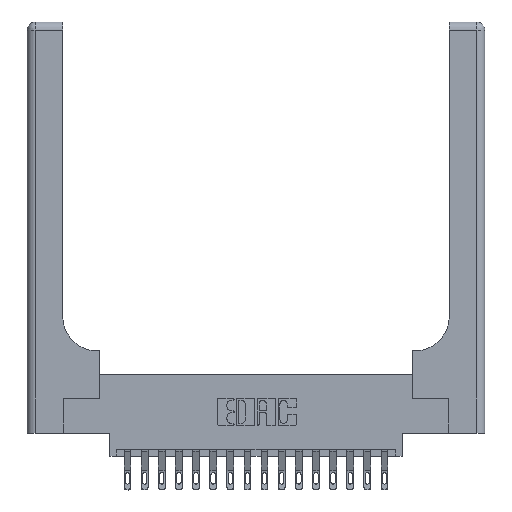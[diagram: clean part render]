
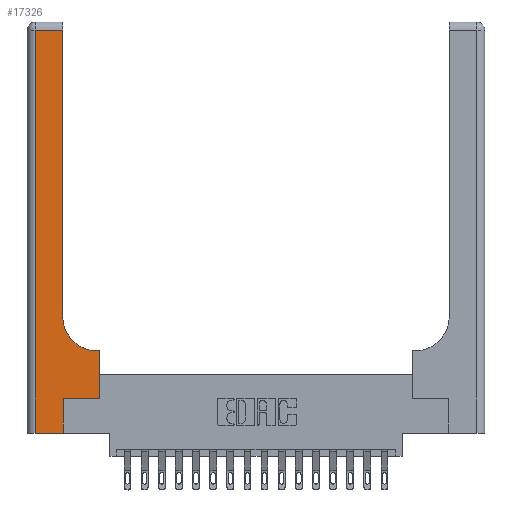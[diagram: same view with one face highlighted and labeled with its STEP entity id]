
A CAD part, top view. The second image highlights one B-rep face of the part: STEP entity #17326.
In plain terms, the highlighted planar face has unit normal (0, 0, 1).
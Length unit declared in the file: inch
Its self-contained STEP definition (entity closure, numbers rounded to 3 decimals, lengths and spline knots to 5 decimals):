
#51 = LINE ( 'NONE', #6856, #16189 ) ;
#417 = ORIENTED_EDGE ( 'NONE', *, *, #19441, .T. ) ;
#775 = EDGE_CURVE ( 'NONE', #4348, #18206, #16440, .T. ) ;
#969 = EDGE_CURVE ( 'NONE', #7376, #7418, #8162, .T. ) ;
#982 = EDGE_LOOP ( 'NONE', ( #9656, #7684, #10253, #3017, #5824, #18833, #3794, #417, #2319 ) ) ;
#1129 = LINE ( 'NONE', #6979, #4694 ) ;
#1224 = DIRECTION ( 'NONE',  ( 0., 0., -1. ) ) ;
#1258 = CARTESIAN_POINT ( 'NONE',  ( 0.528, 0.6, 0.37 ) ) ;
#1745 = EDGE_CURVE ( 'NONE', #18206, #7376, #11112, .T. ) ;
#1883 = DIRECTION ( 'NONE',  ( 1., 0., 0. ) ) ;
#2319 = ORIENTED_EDGE ( 'NONE', *, *, #7392, .T. ) ;
#2387 = VERTEX_POINT ( 'NONE', #19251 ) ;
#2564 = CARTESIAN_POINT ( 'NONE',  ( 0.06, 0., 0.37 ) ) ;
#2622 = LINE ( 'NONE', #18035, #18233 ) ;
#2755 = PLANE ( 'NONE',  #16710 ) ;
#2839 = FACE_OUTER_BOUND ( 'NONE', #982, .T. ) ;
#3017 = ORIENTED_EDGE ( 'NONE', *, *, #775, .T. ) ;
#3207 = DIRECTION ( 'NONE',  ( 0., 1., 0. ) ) ;
#3646 = CARTESIAN_POINT ( 'NONE',  ( 0.265, 0., 0.37 ) ) ;
#3794 = ORIENTED_EDGE ( 'NONE', *, *, #7084, .T. ) ;
#4286 = CARTESIAN_POINT ( 'NONE',  ( 0., 3., 0.37 ) ) ;
#4348 = VERTEX_POINT ( 'NONE', #2564 ) ;
#4694 = VECTOR ( 'NONE', #11569, 39.37008 ) ;
#4829 = EDGE_CURVE ( 'NONE', #9196, #4348, #51, .T. ) ;
#5149 = CARTESIAN_POINT ( 'NONE',  ( 0.51, 0.85, 0.37 ) ) ;
#5661 = CARTESIAN_POINT ( 'NONE',  ( 0.265, 0., 0.37 ) ) ;
#5823 = DIRECTION ( 'NONE',  ( -1., 0., 0. ) ) ;
#5824 = ORIENTED_EDGE ( 'NONE', *, *, #1745, .T. ) ;
#5871 = CARTESIAN_POINT ( 'NONE',  ( 0.06, 2.94, 0.37 ) ) ;
#6522 = CARTESIAN_POINT ( 'NONE',  ( 0.51, 0.6, 0.37 ) ) ;
#6675 = DIRECTION ( 'NONE',  ( 1., 0., 0. ) ) ;
#6856 = CARTESIAN_POINT ( 'NONE',  ( 0.06, 3., 0.37 ) ) ;
#6979 = CARTESIAN_POINT ( 'NONE',  ( 0.26, 0.6, 0.37 ) ) ;
#7084 = EDGE_CURVE ( 'NONE', #7418, #9750, #2622, .T. ) ;
#7252 = CARTESIAN_POINT ( 'NONE',  ( 0., 2.94, 0.37 ) ) ;
#7376 = VERTEX_POINT ( 'NONE', #12654 ) ;
#7392 = EDGE_CURVE ( 'NONE', #11188, #11655, #17981, .T. ) ;
#7418 = VERTEX_POINT ( 'NONE', #11252 ) ;
#7596 = LINE ( 'NONE', #15277, #15171 ) ;
#7684 = ORIENTED_EDGE ( 'NONE', *, *, #17955, .T. ) ;
#7954 = CARTESIAN_POINT ( 'NONE',  ( 0., 0., 0.37 ) ) ;
#8162 = LINE ( 'NONE', #17450, #15729 ) ;
#8340 = VECTOR ( 'NONE', #19336, 39.37008 ) ;
#9196 = VERTEX_POINT ( 'NONE', #5871 ) ;
#9656 = ORIENTED_EDGE ( 'NONE', *, *, #17540, .T. ) ;
#9750 = VERTEX_POINT ( 'NONE', #1258 ) ;
#9940 = DIRECTION ( 'NONE',  ( 1., 0., 0. ) ) ;
#10253 = ORIENTED_EDGE ( 'NONE', *, *, #4829, .T. ) ;
#11112 = LINE ( 'NONE', #5661, #14660 ) ;
#11188 = VERTEX_POINT ( 'NONE', #6522 ) ;
#11252 = CARTESIAN_POINT ( 'NONE',  ( 0.528, 0.25, 0.37 ) ) ;
#11569 = DIRECTION ( 'NONE',  ( -1., 0., 0. ) ) ;
#11655 = VERTEX_POINT ( 'NONE', #15569 ) ;
#12654 = CARTESIAN_POINT ( 'NONE',  ( 0.265, 0.25, 0.37 ) ) ;
#14660 = VECTOR ( 'NONE', #16243, 39.37008 ) ;
#15171 = VECTOR ( 'NONE', #3207, 39.37008 ) ;
#15277 = CARTESIAN_POINT ( 'NONE',  ( 0.26, 3., 0.37 ) ) ;
#15569 = CARTESIAN_POINT ( 'NONE',  ( 0.26, 0.85, 0.37 ) ) ;
#15729 = VECTOR ( 'NONE', #9940, 39.37008 ) ;
#15754 = DIRECTION ( 'NONE',  ( 0., 0., -1. ) ) ;
#16189 = VECTOR ( 'NONE', #18952, 39.37008 ) ;
#16243 = DIRECTION ( 'NONE',  ( 0., 1., 0. ) ) ;
#16363 = LINE ( 'NONE', #7252, #8340 ) ;
#16440 = LINE ( 'NONE', #7954, #19014 ) ;
#16710 = AXIS2_PLACEMENT_3D ( 'NONE', #4286, #1224, #5823 ) ;
#17326 = ADVANCED_FACE ( 'NONE', ( #2839 ), #2755, .F. ) ;
#17450 = CARTESIAN_POINT ( 'NONE',  ( 0.265, 0.25, 0.37 ) ) ;
#17540 = EDGE_CURVE ( 'NONE', #11655, #2387, #7596, .T. ) ;
#17955 = EDGE_CURVE ( 'NONE', #2387, #9196, #16363, .T. ) ;
#17981 = CIRCLE ( 'NONE', #19024, 0.25 ) ;
#18035 = CARTESIAN_POINT ( 'NONE',  ( 0.528, 0.25, 0.37 ) ) ;
#18099 = DIRECTION ( 'NONE',  ( 0., 1., 0. ) ) ;
#18206 = VERTEX_POINT ( 'NONE', #3646 ) ;
#18233 = VECTOR ( 'NONE', #18099, 39.37008 ) ;
#18833 = ORIENTED_EDGE ( 'NONE', *, *, #969, .T. ) ;
#18952 = DIRECTION ( 'NONE',  ( 0., -1., 0. ) ) ;
#19014 = VECTOR ( 'NONE', #1883, 39.37008 ) ;
#19024 = AXIS2_PLACEMENT_3D ( 'NONE', #5149, #15754, #6675 ) ;
#19251 = CARTESIAN_POINT ( 'NONE',  ( 0.26, 2.94, 0.37 ) ) ;
#19336 = DIRECTION ( 'NONE',  ( -1., 0., 0. ) ) ;
#19441 = EDGE_CURVE ( 'NONE', #9750, #11188, #1129, .T. ) ;
